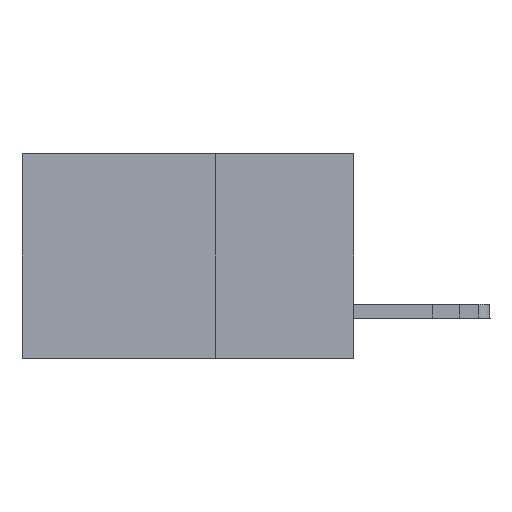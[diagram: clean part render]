
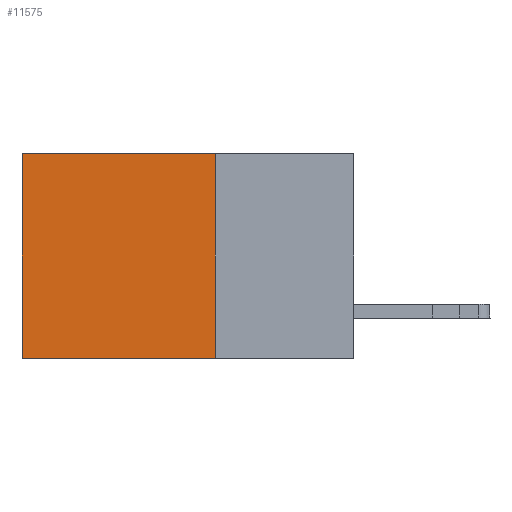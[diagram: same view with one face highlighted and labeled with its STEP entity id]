
A CAD part, left-side view. The second image highlights one B-rep face of the part: STEP entity #11575.
In plain terms, the highlighted planar face has unit normal (-1, 0, 0).
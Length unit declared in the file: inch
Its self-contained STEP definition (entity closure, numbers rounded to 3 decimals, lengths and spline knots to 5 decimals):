
#388 = VECTOR ( 'NONE', #7752, 39.37008 ) ;
#446 = CARTESIAN_POINT ( 'NONE',  ( 0.2875, 0.6, 0. ) ) ;
#563 = EDGE_LOOP ( 'NONE', ( #4456, #2753, #3916, #3580 ) ) ;
#1791 = LINE ( 'NONE', #21247, #388 ) ;
#2315 = DIRECTION ( 'NONE',  ( 1., 0., 0. ) ) ;
#2753 = ORIENTED_EDGE ( 'NONE', *, *, #22967, .F. ) ;
#2758 = DIRECTION ( 'NONE',  ( 0., 0., -1. ) ) ;
#3000 = CARTESIAN_POINT ( 'NONE',  ( 0.2875, 0.25, 0. ) ) ;
#3580 = ORIENTED_EDGE ( 'NONE', *, *, #7979, .T. ) ;
#3916 = ORIENTED_EDGE ( 'NONE', *, *, #20175, .F. ) ;
#4456 = ORIENTED_EDGE ( 'NONE', *, *, #6799, .T. ) ;
#5175 = CARTESIAN_POINT ( 'NONE',  ( 0.2875, 0.25, 0. ) ) ;
#6352 = LINE ( 'NONE', #446, #17773 ) ;
#6799 = EDGE_CURVE ( 'NONE', #17100, #11384, #6352, .T. ) ;
#6891 = FACE_OUTER_BOUND ( 'NONE', #563, .T. ) ;
#7752 = DIRECTION ( 'NONE',  ( 0., 1., 0. ) ) ;
#7979 = EDGE_CURVE ( 'NONE', #8410, #17100, #22858, .T. ) ;
#8410 = VERTEX_POINT ( 'NONE', #13623 ) ;
#11207 = AXIS2_PLACEMENT_3D ( 'NONE', #26949, #2315, #18301 ) ;
#11384 = VERTEX_POINT ( 'NONE', #19735 ) ;
#11575 = ADVANCED_FACE ( 'NONE', ( #6891 ), #18199, .F. ) ;
#13623 = CARTESIAN_POINT ( 'NONE',  ( 0.2875, 0.25, 0. ) ) ;
#17100 = VERTEX_POINT ( 'NONE', #18265 ) ;
#17773 = VECTOR ( 'NONE', #2758, 39.37008 ) ;
#18199 = PLANE ( 'NONE',  #11207 ) ;
#18265 = CARTESIAN_POINT ( 'NONE',  ( 0.2875, 0.6, 0. ) ) ;
#18301 = DIRECTION ( 'NONE',  ( 0., 0., -1. ) ) ;
#19735 = CARTESIAN_POINT ( 'NONE',  ( 0.2875, 0.6, -0.37 ) ) ;
#20175 = EDGE_CURVE ( 'NONE', #8410, #24141, #25954, .T. ) ;
#20187 = VECTOR ( 'NONE', #27429, 39.37008 ) ;
#21247 = CARTESIAN_POINT ( 'NONE',  ( 0.2875, 0.25, -0.37 ) ) ;
#22858 = LINE ( 'NONE', #3000, #28626 ) ;
#22967 = EDGE_CURVE ( 'NONE', #24141, #11384, #1791, .T. ) ;
#24141 = VERTEX_POINT ( 'NONE', #24616 ) ;
#24616 = CARTESIAN_POINT ( 'NONE',  ( 0.2875, 0.25, -0.37 ) ) ;
#25385 = DIRECTION ( 'NONE',  ( 0., 1., 0. ) ) ;
#25954 = LINE ( 'NONE', #5175, #20187 ) ;
#26949 = CARTESIAN_POINT ( 'NONE',  ( 0.2875, 0.25, 0. ) ) ;
#27429 = DIRECTION ( 'NONE',  ( 0., 0., -1. ) ) ;
#28626 = VECTOR ( 'NONE', #25385, 39.37008 ) ;
